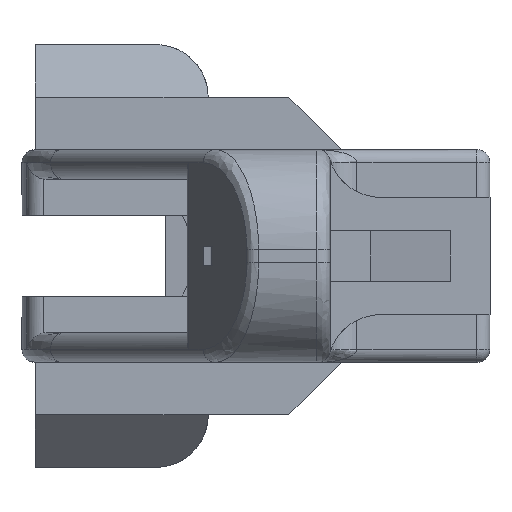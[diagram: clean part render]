
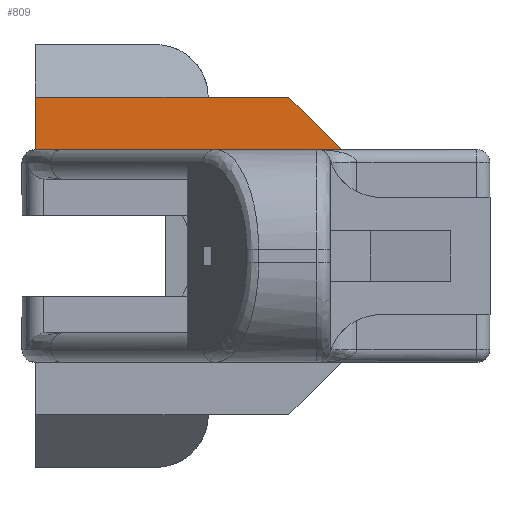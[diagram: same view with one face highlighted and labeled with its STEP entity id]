
A CAD part, left-side view. The second image highlights one B-rep face of the part: STEP entity #809.
In plain terms, the highlighted planar face has unit normal (-1, 0, 0).
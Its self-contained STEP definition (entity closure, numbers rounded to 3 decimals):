
#118 = VERTEX_POINT ( 'NONE', #2476 ) ;
#120 = VERTEX_POINT ( 'NONE', #2466 ) ;
#358 = EDGE_CURVE ( 'NONE', #118, #120, #2630, .T. ) ;
#389 = EDGE_CURVE ( 'NONE', #1350, #118, #2750, .T. ) ;
#419 = EDGE_CURVE ( 'NONE', #120, #1344, #2866, .T. ) ;
#438 = EDGE_CURVE ( 'NONE', #1344, #1370, #2937, .T. ) ;
#444 = EDGE_CURVE ( 'NONE', #1370, #1350, #2943, .T. ) ;
#809 = ADVANCED_FACE ( 'NONE', ( #3713 ), #4884, .F. ) ;
#1344 = VERTEX_POINT ( 'NONE', #6242 ) ;
#1350 = VERTEX_POINT ( 'NONE', #6271 ) ;
#1370 = VERTEX_POINT ( 'NONE', #6290 ) ;
#1583 = EDGE_LOOP ( 'NONE', ( #1713, #1720, #1717, #1759, #1709 ) ) ;
#1709 = ORIENTED_EDGE ( 'NONE', *, *, #389, .T. ) ;
#1713 = ORIENTED_EDGE ( 'NONE', *, *, #358, .T. ) ;
#1717 = ORIENTED_EDGE ( 'NONE', *, *, #438, .T. ) ;
#1720 = ORIENTED_EDGE ( 'NONE', *, *, #419, .T. ) ;
#1759 = ORIENTED_EDGE ( 'NONE', *, *, #444, .T. ) ;
#2466 = CARTESIAN_POINT ( 'NONE',  ( -23.884, -2.114, 40.64 ) ) ;
#2476 = CARTESIAN_POINT ( 'NONE',  ( -23.884, 56.286, 40.64 ) ) ;
#2630 = LINE ( 'NONE', #2645, #6464 ) ;
#2632 = DIRECTION ( 'NONE',  ( 0., -1., 0. ) ) ;
#2645 = CARTESIAN_POINT ( 'NONE',  ( -23.884, 56.286, 40.64 ) ) ;
#2719 = CARTESIAN_POINT ( 'NONE',  ( -23.884, 56.286, 55.64 ) ) ;
#2720 = DIRECTION ( 'NONE',  ( 0., 0., -1. ) ) ;
#2750 = LINE ( 'NONE', #2719, #4018 ) ;
#2866 = LINE ( 'NONE', #2867, #4049 ) ;
#2867 = CARTESIAN_POINT ( 'NONE',  ( -23.884, -2.114, 40.64 ) ) ;
#2868 = DIRECTION ( 'NONE',  ( 0., 0.707, 0.707 ) ) ;
#2911 = CARTESIAN_POINT ( 'NONE',  ( -23.884, -2.114, 50.64 ) ) ;
#2925 = DIRECTION ( 'NONE',  ( 0., 1., 0. ) ) ;
#2937 = LINE ( 'NONE', #2911, #4070 ) ;
#2943 = LINE ( 'NONE', #2947, #4105 ) ;
#2947 = CARTESIAN_POINT ( 'NONE',  ( -23.884, 56.286, 50.64 ) ) ;
#2949 = DIRECTION ( 'NONE',  ( 0., 1., 0. ) ) ;
#3687 = AXIS2_PLACEMENT_3D ( 'NONE', #4876, #4867, #4881 ) ;
#3713 = FACE_OUTER_BOUND ( 'NONE', #1583, .T. ) ;
#4018 = VECTOR ( 'NONE', #2720, 1000. ) ;
#4049 = VECTOR ( 'NONE', #2868, 1000. ) ;
#4070 = VECTOR ( 'NONE', #2925, 1000. ) ;
#4105 = VECTOR ( 'NONE', #2949, 1000. ) ;
#4867 = DIRECTION ( 'NONE',  ( 1., 0., 0. ) ) ;
#4876 = CARTESIAN_POINT ( 'NONE',  ( -23.884, 56.286, 55.64 ) ) ;
#4881 = DIRECTION ( 'NONE',  ( 0., 1., 0. ) ) ;
#4884 = PLANE ( 'NONE',  #3687 ) ;
#6242 = CARTESIAN_POINT ( 'NONE',  ( -23.884, 7.886, 50.64 ) ) ;
#6271 = CARTESIAN_POINT ( 'NONE',  ( -23.884, 56.286, 50.64 ) ) ;
#6290 = CARTESIAN_POINT ( 'NONE',  ( -23.884, 23.286, 50.64 ) ) ;
#6464 = VECTOR ( 'NONE', #2632, 1000. ) ;
